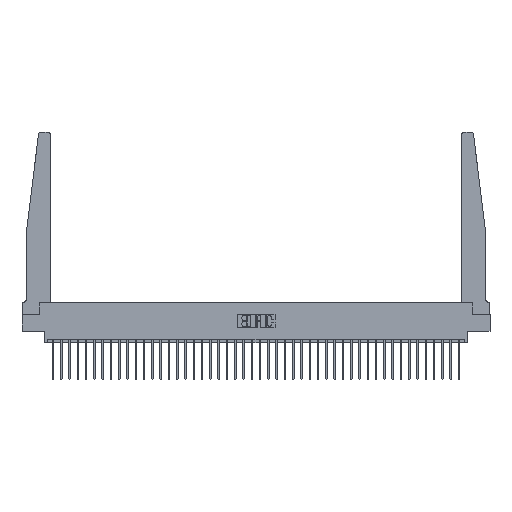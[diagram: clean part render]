
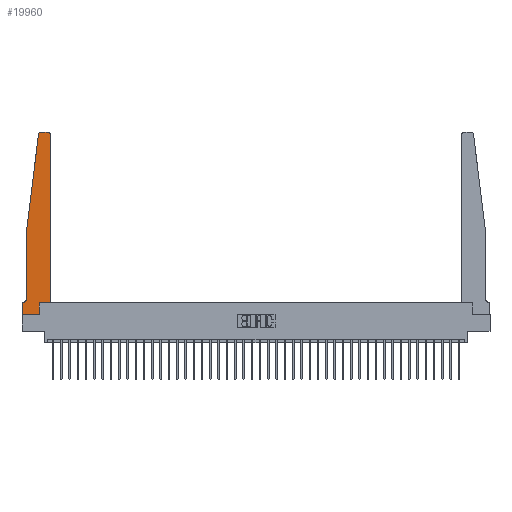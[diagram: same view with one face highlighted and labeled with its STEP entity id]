
A CAD part, top view. The second image highlights one B-rep face of the part: STEP entity #19960.
In plain terms, the highlighted planar face has unit normal (0, 0, 1).
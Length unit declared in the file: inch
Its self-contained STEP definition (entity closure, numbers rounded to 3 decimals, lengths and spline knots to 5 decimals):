
#1138 = CARTESIAN_POINT ( 'NONE',  ( 0.27653, 2.75, 0.37 ) ) ;
#1661 = CARTESIAN_POINT ( 'NONE',  ( 0.065, 1.25, 0.37 ) ) ;
#2264 = VERTEX_POINT ( 'NONE', #24082 ) ;
#2270 = DIRECTION ( 'NONE',  ( 0., 0., 1. ) ) ;
#2507 = DIRECTION ( 'NONE',  ( -1., 0., 0. ) ) ;
#2814 = CARTESIAN_POINT ( 'NONE',  ( 0.2605, 0.18, 0.37 ) ) ;
#2834 = VECTOR ( 'NONE', #6910, 39.37008 ) ;
#3003 = DIRECTION ( 'NONE',  ( 1., 0., 0. ) ) ;
#3527 = AXIS2_PLACEMENT_3D ( 'NONE', #13768, #36567, #22366 ) ;
#3575 = VECTOR ( 'NONE', #31360, 39.37008 ) ;
#3807 = ORIENTED_EDGE ( 'NONE', *, *, #15051, .T. ) ;
#3891 = CARTESIAN_POINT ( 'NONE',  ( 0.065, 0.2375, 0.37 ) ) ;
#4787 = CARTESIAN_POINT ( 'NONE',  ( 0.065, 1.25, 0.37 ) ) ;
#5627 = CARTESIAN_POINT ( 'NONE',  ( 0.25, 2.75, 0.37 ) ) ;
#5795 = LINE ( 'NONE', #28434, #33781 ) ;
#5922 = EDGE_CURVE ( 'NONE', #35441, #12894, #36512, .T. ) ;
#5994 = CARTESIAN_POINT ( 'NONE',  ( 0.395, 2.75, 0.37 ) ) ;
#6910 = DIRECTION ( 'NONE',  ( -0.122, -0.992, 0. ) ) ;
#7876 = FACE_OUTER_BOUND ( 'NONE', #26176, .T. ) ;
#8374 = DIRECTION ( 'NONE',  ( 0., 0., 1. ) ) ;
#8875 = EDGE_CURVE ( 'NONE', #10872, #34841, #5795, .T. ) ;
#8934 = VERTEX_POINT ( 'NONE', #14785 ) ;
#9411 = CARTESIAN_POINT ( 'NONE',  ( 0.2605, 0., 0.37 ) ) ;
#9677 = VECTOR ( 'NONE', #10879, 39.37008 ) ;
#10872 = VERTEX_POINT ( 'NONE', #14002 ) ;
#10879 = DIRECTION ( 'NONE',  ( -1., 0., 0. ) ) ;
#11674 = CARTESIAN_POINT ( 'NONE',  ( 0.425, 0.18, 0.37 ) ) ;
#11928 = CARTESIAN_POINT ( 'NONE',  ( 0.24675, 2.72367, 0.37 ) ) ;
#12237 = VECTOR ( 'NONE', #17673, 39.37008 ) ;
#12551 = EDGE_CURVE ( 'NONE', #14698, #16050, #26546, .T. ) ;
#12894 = VERTEX_POINT ( 'NONE', #13185 ) ;
#13057 = AXIS2_PLACEMENT_3D ( 'NONE', #17166, #8374, #16800 ) ;
#13185 = CARTESIAN_POINT ( 'NONE',  ( 0., 0.1875, 0.37 ) ) ;
#13186 = ORIENTED_EDGE ( 'NONE', *, *, #17956, .T. ) ;
#13353 = ORIENTED_EDGE ( 'NONE', *, *, #36026, .T. ) ;
#13508 = LINE ( 'NONE', #5627, #9677 ) ;
#13570 = ORIENTED_EDGE ( 'NONE', *, *, #5922, .T. ) ;
#13684 = DIRECTION ( 'NONE',  ( 1., 0., 0. ) ) ;
#13768 = CARTESIAN_POINT ( 'NONE',  ( 0.395, 2.72, 0.37 ) ) ;
#14002 = CARTESIAN_POINT ( 'NONE',  ( 0., 0., 0.37 ) ) ;
#14513 = ORIENTED_EDGE ( 'NONE', *, *, #25090, .T. ) ;
#14698 = VERTEX_POINT ( 'NONE', #11928 ) ;
#14785 = CARTESIAN_POINT ( 'NONE',  ( 0.2605, 0.18, 0.37 ) ) ;
#15051 = EDGE_CURVE ( 'NONE', #30325, #33408, #19081, .T. ) ;
#15791 = ORIENTED_EDGE ( 'NONE', *, *, #33351, .T. ) ;
#16050 = VERTEX_POINT ( 'NONE', #4787 ) ;
#16054 = LINE ( 'NONE', #1661, #33104 ) ;
#16800 = DIRECTION ( 'NONE',  ( 1., 0., 0. ) ) ;
#17030 = EDGE_CURVE ( 'NONE', #34841, #8934, #33678, .T. ) ;
#17166 = CARTESIAN_POINT ( 'NONE',  ( 0.27653, 2.72, 0.37 ) ) ;
#17505 = DIRECTION ( 'NONE',  ( 0., -1., 0. ) ) ;
#17673 = DIRECTION ( 'NONE',  ( 1., 0., 0. ) ) ;
#17956 = EDGE_CURVE ( 'NONE', #35792, #35441, #20425, .T. ) ;
#19054 = DIRECTION ( 'NONE',  ( 0., -1., 0. ) ) ;
#19081 = CIRCLE ( 'NONE', #3527, 0.03 ) ;
#19114 = EDGE_CURVE ( 'NONE', #12894, #10872, #23107, .T. ) ;
#19773 = VECTOR ( 'NONE', #24902, 39.37008 ) ;
#19820 = AXIS2_PLACEMENT_3D ( 'NONE', #28127, #22700, #2507 ) ;
#19960 = ADVANCED_FACE ( 'NONE', ( #7876 ), #24715, .T. ) ;
#19969 = LINE ( 'NONE', #34732, #3575 ) ;
#20425 = CIRCLE ( 'NONE', #19820, 0.05 ) ;
#21132 = CARTESIAN_POINT ( 'NONE',  ( 0.065, 1.25, 0.37 ) ) ;
#22177 = ORIENTED_EDGE ( 'NONE', *, *, #36665, .T. ) ;
#22366 = DIRECTION ( 'NONE',  ( 1., 0., 0. ) ) ;
#22408 = VECTOR ( 'NONE', #17505, 39.37008 ) ;
#22700 = DIRECTION ( 'NONE',  ( 0., 0., -1. ) ) ;
#23107 = LINE ( 'NONE', #34508, #22408 ) ;
#23466 = ORIENTED_EDGE ( 'NONE', *, *, #12551, .T. ) ;
#23827 = LINE ( 'NONE', #11674, #12237 ) ;
#23842 = EDGE_CURVE ( 'NONE', #29777, #14698, #29175, .T. ) ;
#23913 = CARTESIAN_POINT ( 'NONE',  ( 0.015, 0.1875, 0.37 ) ) ;
#24082 = CARTESIAN_POINT ( 'NONE',  ( 0.425, 0.18, 0.37 ) ) ;
#24715 = PLANE ( 'NONE',  #32553 ) ;
#24902 = DIRECTION ( 'NONE',  ( 0., 1., 0. ) ) ;
#25090 = EDGE_CURVE ( 'NONE', #2264, #30325, #19969, .T. ) ;
#25529 = ORIENTED_EDGE ( 'NONE', *, *, #19114, .T. ) ;
#26176 = EDGE_LOOP ( 'NONE', ( #15791, #32856, #23466, #13353, #13186, #13570, #25529, #31704, #29673, #22177, #14513, #3807 ) ) ;
#26546 = LINE ( 'NONE', #21132, #2834 ) ;
#27893 = CARTESIAN_POINT ( 'NONE',  ( 0., 0.1875, 0.37 ) ) ;
#28127 = CARTESIAN_POINT ( 'NONE',  ( 0.015, 0.2375, 0.37 ) ) ;
#28434 = CARTESIAN_POINT ( 'NONE',  ( 0., 0., 0.37 ) ) ;
#29175 = CIRCLE ( 'NONE', #13057, 0.03 ) ;
#29673 = ORIENTED_EDGE ( 'NONE', *, *, #17030, .T. ) ;
#29777 = VERTEX_POINT ( 'NONE', #1138 ) ;
#30074 = VECTOR ( 'NONE', #32783, 39.37008 ) ;
#30325 = VERTEX_POINT ( 'NONE', #33238 ) ;
#31360 = DIRECTION ( 'NONE',  ( 0., 1., 0. ) ) ;
#31704 = ORIENTED_EDGE ( 'NONE', *, *, #8875, .T. ) ;
#32553 = AXIS2_PLACEMENT_3D ( 'NONE', #27893, #2270, #13684 ) ;
#32783 = DIRECTION ( 'NONE',  ( -1., 0., 0. ) ) ;
#32856 = ORIENTED_EDGE ( 'NONE', *, *, #23842, .T. ) ;
#33104 = VECTOR ( 'NONE', #19054, 39.37008 ) ;
#33238 = CARTESIAN_POINT ( 'NONE',  ( 0.425, 2.72, 0.37 ) ) ;
#33333 = CARTESIAN_POINT ( 'NONE',  ( 0.065, 0.1875, 0.37 ) ) ;
#33351 = EDGE_CURVE ( 'NONE', #33408, #29777, #13508, .T. ) ;
#33408 = VERTEX_POINT ( 'NONE', #5994 ) ;
#33678 = LINE ( 'NONE', #2814, #19773 ) ;
#33781 = VECTOR ( 'NONE', #3003, 39.37008 ) ;
#34508 = CARTESIAN_POINT ( 'NONE',  ( 0., 0., 0.37 ) ) ;
#34732 = CARTESIAN_POINT ( 'NONE',  ( 0.425, 0.18, 0.37 ) ) ;
#34841 = VERTEX_POINT ( 'NONE', #9411 ) ;
#35441 = VERTEX_POINT ( 'NONE', #23913 ) ;
#35792 = VERTEX_POINT ( 'NONE', #3891 ) ;
#36026 = EDGE_CURVE ( 'NONE', #16050, #35792, #16054, .T. ) ;
#36512 = LINE ( 'NONE', #33333, #30074 ) ;
#36567 = DIRECTION ( 'NONE',  ( 0., 0., 1. ) ) ;
#36665 = EDGE_CURVE ( 'NONE', #8934, #2264, #23827, .T. ) ;
